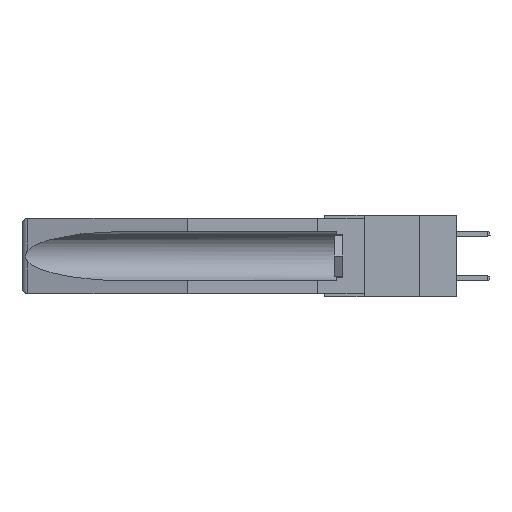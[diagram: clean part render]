
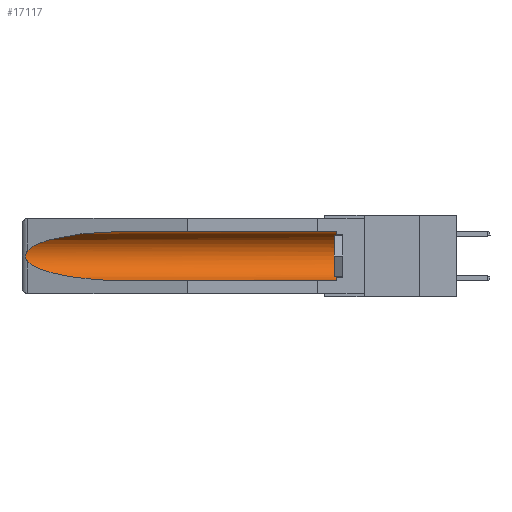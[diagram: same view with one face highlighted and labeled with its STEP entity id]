
A CAD part, left-side view. The second image highlights one B-rep face of the part: STEP entity #17117.
In plain terms, the highlighted cylindrical face has radius 2.857 mm (diameter 5.715 mm), a partial arc.
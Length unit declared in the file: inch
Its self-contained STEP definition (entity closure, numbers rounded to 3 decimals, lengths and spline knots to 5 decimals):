
#35 = CARTESIAN_POINT ( 'NONE',  ( 0.155, 0.126, -0.059 ) ) ;
#436 = CARTESIAN_POINT ( 'NONE',  ( 0.2673, 1.5327, -0.16383 ) ) ;
#501 = CARTESIAN_POINT ( 'NONE',  ( 0.26537, 1.52718, -0.14972 ) ) ;
#579 = CARTESIAN_POINT ( 'NONE',  ( 0.2673, 1.53269, -0.17917 ) ) ;
#647 = VERTEX_POINT ( 'NONE', #8653 ) ;
#764 = CARTESIAN_POINT ( 'NONE',  ( 0.25451, 1.48313, -0.09465 ) ) ;
#2176 = CARTESIAN_POINT ( 'NONE',  ( 0.26537, 1.52718, -0.19328 ) ) ;
#2211 = CARTESIAN_POINT ( 'NONE',  ( 0.26537, 1.52718, -0.19328 ) ) ;
#3241 = VERTEX_POINT ( 'NONE', #2176 ) ;
#3343 = VERTEX_POINT ( 'NONE', #10622 ) ;
#3616 = CARTESIAN_POINT ( 'NONE',  ( 0.2675, 1.53308, -0.17534 ) ) ;
#4100 = DIRECTION ( 'NONE',  ( 0., 0., 1. ) ) ;
#4241 = CARTESIAN_POINT ( 'NONE',  ( 0.155, 0.126, -0.1715 ) ) ;
#4721 = CARTESIAN_POINT ( 'NONE',  ( 0.26537, 1.52718, -0.19328 ) ) ;
#5300 = ORIENTED_EDGE ( 'NONE', *, *, #16241, .T. ) ;
#5493 = CARTESIAN_POINT ( 'NONE',  ( 0.26537, 1.52718, -0.14972 ) ) ;
#5735 = CARTESIAN_POINT ( 'NONE',  ( 0.155, 1.07973, -0.284 ) ) ;
#5763 = DIRECTION ( 'NONE',  ( 0., 1., 0. ) ) ;
#5925 = AXIS2_PLACEMENT_3D ( 'NONE', #20769, #7993, #12867 ) ;
#6502 = ORIENTED_EDGE ( 'NONE', *, *, #12353, .T. ) ;
#6901 = CIRCLE ( 'NONE', #12478, 0.1125 ) ;
#7294 = CARTESIAN_POINT ( 'NONE',  ( 0.155, 1.07973, -0.059 ) ) ;
#7302 = CARTESIAN_POINT ( 'NONE',  ( 0.155, -0.30754, -0.059 ) ) ;
#7941 = EDGE_CURVE ( 'NONE', #3343, #647, #17801, .T. ) ;
#7993 = DIRECTION ( 'NONE',  ( 0., 1., 0. ) ) ;
#8008 = CARTESIAN_POINT ( 'NONE',  ( 0.155, 1.07973, -0.284 ) ) ;
#8246 = EDGE_CURVE ( 'NONE', #3241, #9480, #14035, .T. ) ;
#8454 = B_SPLINE_CURVE_WITH_KNOTS ( 'NONE', 3,
 ( #501, #19972, #10313, #436, #11717, #3616, #579, #18220, #11930, #2211 ),
 .UNSPECIFIED., .F., .F.,
 ( 4, 2, 2, 2, 4 ),
 ( 0., 0.00029, 0.00058, 0.00087, 0.00117 ),
 .UNSPECIFIED. ) ;
#8653 = CARTESIAN_POINT ( 'NONE',  ( 0.26537, 1.52718, -0.14972 ) ) ;
#9159 = DIRECTION ( 'NONE',  ( 0., -1., 0. ) ) ;
#9480 = VERTEX_POINT ( 'NONE', #5735 ) ;
#9676 = ORIENTED_EDGE ( 'NONE', *, *, #8246, .T. ) ;
#9862 = VECTOR ( 'NONE', #10591, 39.37008 ) ;
#10256 = VERTEX_POINT ( 'NONE', #35 ) ;
#10267 = EDGE_LOOP ( 'NONE', ( #20503, #19132, #9676, #14719, #5300, #6502 ) ) ;
#10313 = CARTESIAN_POINT ( 'NONE',  ( 0.26654, 1.53092, -0.15636 ) ) ;
#10421 = VERTEX_POINT ( 'NONE', #11602 ) ;
#10591 = DIRECTION ( 'NONE',  ( 0., 1., 0. ) ) ;
#10622 = CARTESIAN_POINT ( 'NONE',  ( 0.155, 1.07973, -0.059 ) ) ;
#11602 = CARTESIAN_POINT ( 'NONE',  ( 0.155, 0.126, -0.284 ) ) ;
#11717 = CARTESIAN_POINT ( 'NONE',  ( 0.2675, 1.53308, -0.16763 ) ) ;
#11930 = CARTESIAN_POINT ( 'NONE',  ( 0.26597, 1.5296, -0.19026 ) ) ;
#12353 = EDGE_CURVE ( 'NONE', #10256, #3343, #19452, .T. ) ;
#12478 = AXIS2_PLACEMENT_3D ( 'NONE', #4241, #9159, #4100 ) ;
#12867 = DIRECTION ( 'NONE',  ( 0., 0., 1. ) ) ;
#12952 = FACE_OUTER_BOUND ( 'NONE', #10267, .T. ) ;
#13812 = CARTESIAN_POINT ( 'NONE',  ( 0.21114, 1.30732, -0.059 ) ) ;
#14035 =( BOUNDED_CURVE ( )  B_SPLINE_CURVE ( 3, ( #4721, #14508, #17686, #8008 ),
 .UNSPECIFIED., .F., .F. ) 
 B_SPLINE_CURVE_WITH_KNOTS ( ( 4, 4 ),
 ( 0.1948, 1.5708 ),
 .UNSPECIFIED. ) 
 CURVE ( )  GEOMETRIC_REPRESENTATION_ITEM ( )  RATIONAL_B_SPLINE_CURVE ( ( 1., 0.848, 0.848, 1. ) ) 
 REPRESENTATION_ITEM ( '' )  );
#14508 = CARTESIAN_POINT ( 'NONE',  ( 0.25451, 1.48313, -0.24835 ) ) ;
#14719 = ORIENTED_EDGE ( 'NONE', *, *, #14854, .F. ) ;
#14854 = EDGE_CURVE ( 'NONE', #10421, #9480, #16609, .T. ) ;
#15731 = CYLINDRICAL_SURFACE ( 'NONE', #5925, 0.1125 ) ;
#16241 = EDGE_CURVE ( 'NONE', #10421, #10256, #6901, .T. ) ;
#16609 = LINE ( 'NONE', #18334, #20391 ) ;
#17117 = ADVANCED_FACE ( 'NONE', ( #12952 ), #15731, .F. ) ;
#17686 = CARTESIAN_POINT ( 'NONE',  ( 0.21114, 1.30732, -0.284 ) ) ;
#17801 =( BOUNDED_CURVE ( )  B_SPLINE_CURVE ( 3, ( #7294, #13812, #764, #5493 ),
 .UNSPECIFIED., .F., .F. ) 
 B_SPLINE_CURVE_WITH_KNOTS ( ( 4, 4 ),
 ( 4.71239, 6.08839 ),
 .UNSPECIFIED. ) 
 CURVE ( )  GEOMETRIC_REPRESENTATION_ITEM ( )  RATIONAL_B_SPLINE_CURVE ( ( 1., 0.848, 0.848, 1. ) ) 
 REPRESENTATION_ITEM ( '' )  );
#18220 = CARTESIAN_POINT ( 'NONE',  ( 0.26655, 1.53094, -0.18657 ) ) ;
#18334 = CARTESIAN_POINT ( 'NONE',  ( 0.155, -0.30754, -0.284 ) ) ;
#19132 = ORIENTED_EDGE ( 'NONE', *, *, #19387, .T. ) ;
#19387 = EDGE_CURVE ( 'NONE', #647, #3241, #8454, .T. ) ;
#19452 = LINE ( 'NONE', #7302, #9862 ) ;
#19972 = CARTESIAN_POINT ( 'NONE',  ( 0.26597, 1.52961, -0.15275 ) ) ;
#20391 = VECTOR ( 'NONE', #5763, 39.37008 ) ;
#20503 = ORIENTED_EDGE ( 'NONE', *, *, #7941, .T. ) ;
#20769 = CARTESIAN_POINT ( 'NONE',  ( 0.155, -0.30754, -0.1715 ) ) ;
